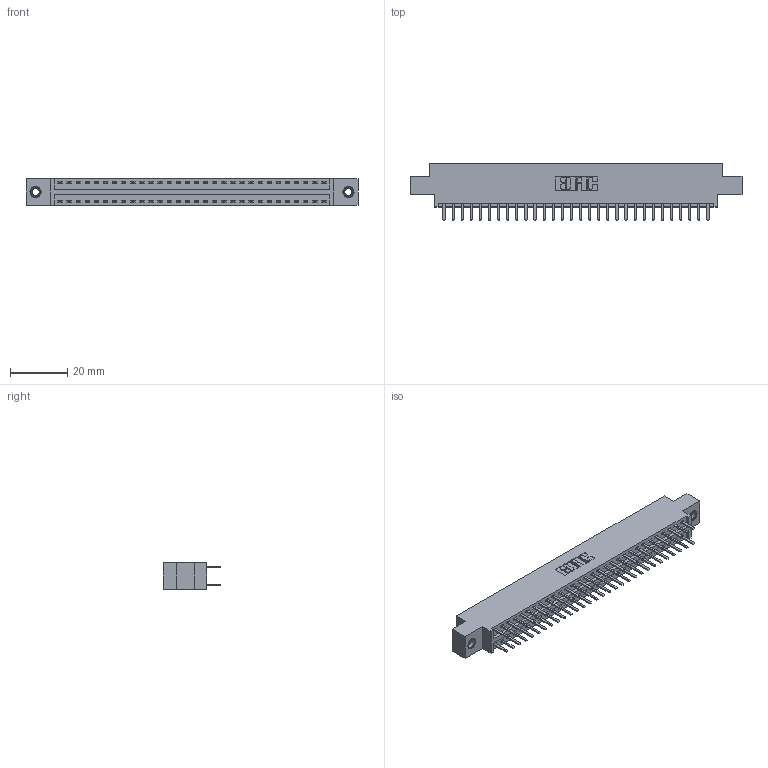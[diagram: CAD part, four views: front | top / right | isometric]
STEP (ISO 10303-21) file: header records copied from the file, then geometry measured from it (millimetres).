
FILE_DESCRIPTION (( 'STEP AP203' ), '1' );
FILE_NAME ('396-060-520-807.STEP', '2019-11-02T08:52:13', ( '' ), ( '' ), 'SwSTEP 2.0', 'SolidWorks 2016', '' );
FILE_SCHEMA (( 'CONFIG_CONTROL_DESIGN' ));
Length unit declared in the file: inch
Products named in the file (4): 346 Part_0.170 Offset - 0.156 Dia-TI; 345-292-001_345-293-120; 345-250-001_345-250-005-103; 396-060-520-807
Assembly tree (63 placements, depth 2):
  396-060-520-807
    346 Part_0.170 Offset - 0.156 Dia-TI
    345-292-001_345-293-120  x60
    345-250-001_345-250-005-103  x2
Bounding box: 115.82 x 20.02 x 9.4 mm (x, y, z)
Volume: 11006.6 mm3; surface area: 15092.2 mm2
Topology: 63 solids, 63 shells, 3546 faces, 10257 edges, 6670 vertices
Faces by surface type: plane 2332, cylinder 1198, cone 12, torus 4
Entity records: 22626 total; most frequent: CARTESIAN_POINT 3743, ORIENTED_EDGE 3658, DIRECTION 3363, EDGE_CURVE 1829, VECTOR 1553, LINE 1553, VERTEX_POINT 1212, AXIS2_PLACEMENT_3D 905
